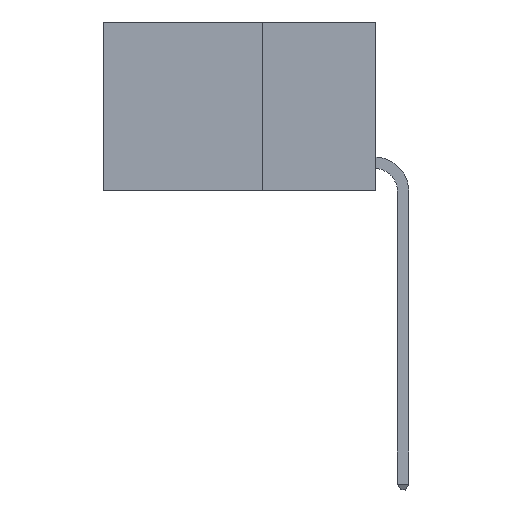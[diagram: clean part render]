
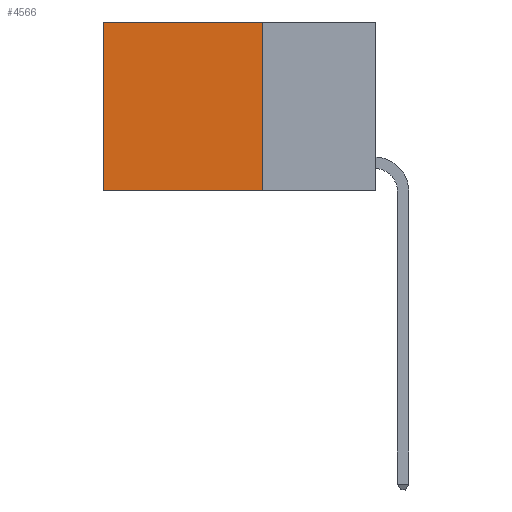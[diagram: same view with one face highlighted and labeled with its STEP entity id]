
A CAD part, left-side view. The second image highlights one B-rep face of the part: STEP entity #4566.
In plain terms, the highlighted planar face has unit normal (-1, 0, 0).
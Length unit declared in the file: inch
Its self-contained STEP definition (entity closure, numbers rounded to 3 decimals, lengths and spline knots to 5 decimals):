
#858 = EDGE_CURVE ( 'NONE', #10812, #12520, #4392, .T. ) ;
#972 = CARTESIAN_POINT ( 'NONE',  ( 0.2625, 0.6, -0.37 ) ) ;
#1282 = CARTESIAN_POINT ( 'NONE',  ( 0.2625, 0.25, -0.37 ) ) ;
#2048 = DIRECTION ( 'NONE',  ( 1., 0., 0. ) ) ;
#2158 = CARTESIAN_POINT ( 'NONE',  ( 0.2625, 0.6, 0. ) ) ;
#2698 = EDGE_LOOP ( 'NONE', ( #8237, #13553, #12550, #12939 ) ) ;
#2918 = CARTESIAN_POINT ( 'NONE',  ( 0.2625, 0.25, -0.37 ) ) ;
#2979 = CARTESIAN_POINT ( 'NONE',  ( 0.2625, 0.6, 0. ) ) ;
#4392 = LINE ( 'NONE', #1282, #6686 ) ;
#4566 = ADVANCED_FACE ( 'NONE', ( #5168 ), #8901, .F. ) ;
#5168 = FACE_OUTER_BOUND ( 'NONE', #2698, .T. ) ;
#5634 = CARTESIAN_POINT ( 'NONE',  ( 0.2625, 0.25, 0. ) ) ;
#6005 = DIRECTION ( 'NONE',  ( 0., 1., 0. ) ) ;
#6029 = CARTESIAN_POINT ( 'NONE',  ( 0.2625, 0.25, 0. ) ) ;
#6446 = DIRECTION ( 'NONE',  ( 0., 0., -1. ) ) ;
#6686 = VECTOR ( 'NONE', #8813, 39.37008 ) ;
#7024 = EDGE_CURVE ( 'NONE', #8453, #12520, #7590, .T. ) ;
#7180 = DIRECTION ( 'NONE',  ( 0., 0., -1. ) ) ;
#7590 = LINE ( 'NONE', #2979, #11758 ) ;
#7774 = LINE ( 'NONE', #13820, #10390 ) ;
#8237 = ORIENTED_EDGE ( 'NONE', *, *, #7024, .T. ) ;
#8453 = VERTEX_POINT ( 'NONE', #2158 ) ;
#8520 = EDGE_CURVE ( 'NONE', #13121, #8453, #7774, .T. ) ;
#8813 = DIRECTION ( 'NONE',  ( 0., 1., 0. ) ) ;
#8901 = PLANE ( 'NONE',  #11698 ) ;
#10013 = DIRECTION ( 'NONE',  ( 0., 0., -1. ) ) ;
#10390 = VECTOR ( 'NONE', #6005, 39.37008 ) ;
#10812 = VERTEX_POINT ( 'NONE', #2918 ) ;
#10901 = EDGE_CURVE ( 'NONE', #13121, #10812, #12389, .T. ) ;
#11698 = AXIS2_PLACEMENT_3D ( 'NONE', #12194, #2048, #10013 ) ;
#11758 = VECTOR ( 'NONE', #6446, 39.37008 ) ;
#12045 = VECTOR ( 'NONE', #7180, 39.37008 ) ;
#12194 = CARTESIAN_POINT ( 'NONE',  ( 0.2625, 0.25, 0. ) ) ;
#12389 = LINE ( 'NONE', #6029, #12045 ) ;
#12520 = VERTEX_POINT ( 'NONE', #972 ) ;
#12550 = ORIENTED_EDGE ( 'NONE', *, *, #10901, .F. ) ;
#12939 = ORIENTED_EDGE ( 'NONE', *, *, #8520, .T. ) ;
#13121 = VERTEX_POINT ( 'NONE', #5634 ) ;
#13553 = ORIENTED_EDGE ( 'NONE', *, *, #858, .F. ) ;
#13820 = CARTESIAN_POINT ( 'NONE',  ( 0.2625, 0.25, 0. ) ) ;
